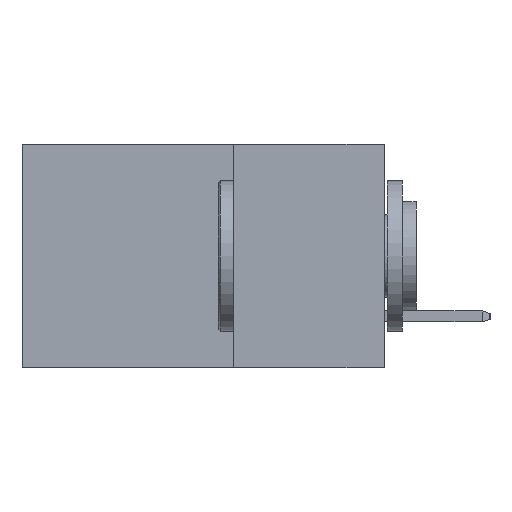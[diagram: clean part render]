
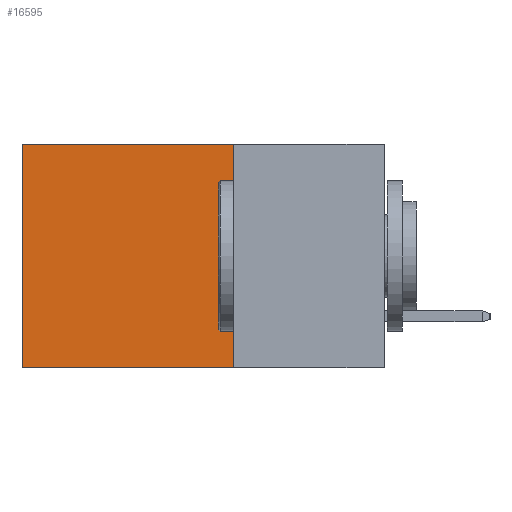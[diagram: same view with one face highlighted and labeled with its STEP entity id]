
A CAD part, left-side view. The second image highlights one B-rep face of the part: STEP entity #16595.
In plain terms, the highlighted planar face has unit normal (-1, 0, 0).
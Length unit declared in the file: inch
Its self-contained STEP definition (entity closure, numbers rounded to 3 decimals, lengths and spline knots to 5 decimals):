
#546 = VECTOR ( 'NONE', #15994, 39.37008 ) ;
#1431 = EDGE_CURVE ( 'NONE', #12347, #13245, #5235, .T. ) ;
#1972 = ORIENTED_EDGE ( 'NONE', *, *, #3553, .F. ) ;
#3553 = EDGE_CURVE ( 'NONE', #12347, #17850, #20800, .T. ) ;
#3632 = CARTESIAN_POINT ( 'NONE',  ( 0.2615, 0.25, -0.37 ) ) ;
#4088 = FACE_OUTER_BOUND ( 'NONE', #14566, .T. ) ;
#4519 = EDGE_CURVE ( 'NONE', #13245, #6128, #9754, .T. ) ;
#5235 = LINE ( 'NONE', #10678, #546 ) ;
#6128 = VERTEX_POINT ( 'NONE', #16497 ) ;
#7302 = VECTOR ( 'NONE', #16184, 39.37008 ) ;
#7977 = CARTESIAN_POINT ( 'NONE',  ( 0.2615, 0.25, -0.37 ) ) ;
#9197 = VECTOR ( 'NONE', #17415, 39.37008 ) ;
#9754 = LINE ( 'NONE', #17471, #9197 ) ;
#10114 = CARTESIAN_POINT ( 'NONE',  ( 0.2615, 0.25, 0. ) ) ;
#10678 = CARTESIAN_POINT ( 'NONE',  ( 0.2615, 0.25, 0. ) ) ;
#12347 = VERTEX_POINT ( 'NONE', #10114 ) ;
#12534 = ORIENTED_EDGE ( 'NONE', *, *, #4519, .T. ) ;
#12908 = CARTESIAN_POINT ( 'NONE',  ( 0.2615, 0.6, 0. ) ) ;
#13245 = VERTEX_POINT ( 'NONE', #12908 ) ;
#14566 = EDGE_LOOP ( 'NONE', ( #12534, #15301, #1972, #20436 ) ) ;
#15301 = ORIENTED_EDGE ( 'NONE', *, *, #20450, .F. ) ;
#15601 = LINE ( 'NONE', #19147, #20443 ) ;
#15994 = DIRECTION ( 'NONE',  ( 0., 1., 0. ) ) ;
#16184 = DIRECTION ( 'NONE',  ( 0., 0., -1. ) ) ;
#16327 = AXIS2_PLACEMENT_3D ( 'NONE', #18868, #18843, #18796 ) ;
#16497 = CARTESIAN_POINT ( 'NONE',  ( 0.2615, 0.6, -0.37 ) ) ;
#16595 = ADVANCED_FACE ( 'NONE', ( #4088 ), #19194, .F. ) ;
#17415 = DIRECTION ( 'NONE',  ( 0., 0., -1. ) ) ;
#17471 = CARTESIAN_POINT ( 'NONE',  ( 0.2615, 0.6, -0.37 ) ) ;
#17850 = VERTEX_POINT ( 'NONE', #3632 ) ;
#18796 = DIRECTION ( 'NONE',  ( 0., 0., -1. ) ) ;
#18843 = DIRECTION ( 'NONE',  ( 1., 0., 0. ) ) ;
#18868 = CARTESIAN_POINT ( 'NONE',  ( 0.2615, 0.25, -0.37 ) ) ;
#19076 = DIRECTION ( 'NONE',  ( 0., 1., 0. ) ) ;
#19147 = CARTESIAN_POINT ( 'NONE',  ( 0.2615, 0.25, -0.37 ) ) ;
#19194 = PLANE ( 'NONE',  #16327 ) ;
#20436 = ORIENTED_EDGE ( 'NONE', *, *, #1431, .T. ) ;
#20443 = VECTOR ( 'NONE', #19076, 39.37008 ) ;
#20450 = EDGE_CURVE ( 'NONE', #17850, #6128, #15601, .T. ) ;
#20800 = LINE ( 'NONE', #7977, #7302 ) ;
